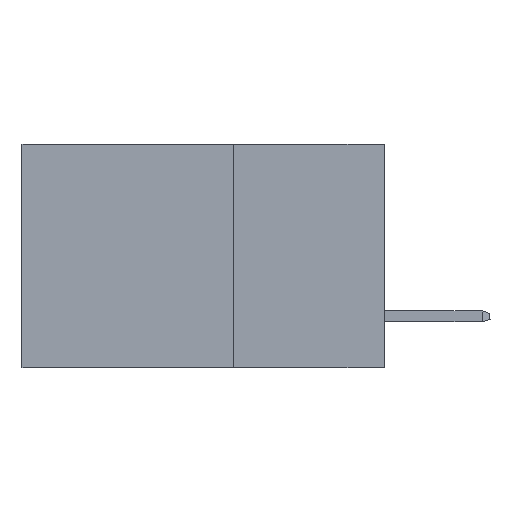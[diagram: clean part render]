
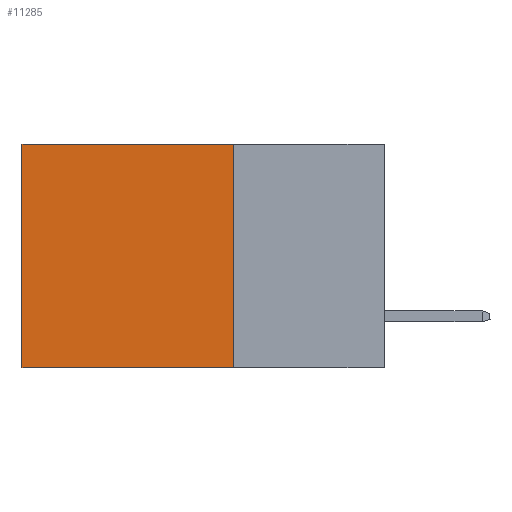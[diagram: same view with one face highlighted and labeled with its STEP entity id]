
A CAD part, left-side view. The second image highlights one B-rep face of the part: STEP entity #11285.
In plain terms, the highlighted planar face has unit normal (-1, 0, 0).
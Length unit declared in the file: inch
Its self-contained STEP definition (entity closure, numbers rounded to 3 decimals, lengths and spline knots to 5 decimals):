
#1179 = ORIENTED_EDGE ( 'NONE', *, *, #7643, .F. ) ;
#1474 = EDGE_CURVE ( 'NONE', #23829, #23262, #9127, .T. ) ;
#2188 = CARTESIAN_POINT ( 'NONE',  ( 0.2615, 0.6, 0. ) ) ;
#2611 = LINE ( 'NONE', #17897, #23378 ) ;
#3363 = DIRECTION ( 'NONE',  ( 0., 0., -1. ) ) ;
#6146 = DIRECTION ( 'NONE',  ( 0., 0., -1. ) ) ;
#7643 = EDGE_CURVE ( 'NONE', #25616, #23262, #22868, .T. ) ;
#8002 = DIRECTION ( 'NONE',  ( 0., 1., 0. ) ) ;
#8077 = CARTESIAN_POINT ( 'NONE',  ( 0.2615, 0.25, -0.37 ) ) ;
#8276 = CARTESIAN_POINT ( 'NONE',  ( 0.2615, 0.6, -0.37 ) ) ;
#9127 = LINE ( 'NONE', #19119, #25031 ) ;
#10938 = CARTESIAN_POINT ( 'NONE',  ( 0.2615, 0.25, -0.37 ) ) ;
#10996 = CARTESIAN_POINT ( 'NONE',  ( 0.2615, 0.25, 0. ) ) ;
#11285 = ADVANCED_FACE ( 'NONE', ( #23899 ), #14159, .F. ) ;
#11448 = CARTESIAN_POINT ( 'NONE',  ( 0.2615, 0.25, -0.37 ) ) ;
#11860 = AXIS2_PLACEMENT_3D ( 'NONE', #8077, #18147, #6146 ) ;
#12409 = DIRECTION ( 'NONE',  ( 0., 1., 0. ) ) ;
#12574 = CARTESIAN_POINT ( 'NONE',  ( 0.2615, 0.25, -0.37 ) ) ;
#12931 = LINE ( 'NONE', #11448, #22915 ) ;
#13049 = EDGE_CURVE ( 'NONE', #24311, #23829, #2611, .T. ) ;
#14060 = ORIENTED_EDGE ( 'NONE', *, *, #1474, .T. ) ;
#14159 = PLANE ( 'NONE',  #11860 ) ;
#17518 = VECTOR ( 'NONE', #12409, 39.37008 ) ;
#17739 = EDGE_LOOP ( 'NONE', ( #14060, #1179, #20037, #19972 ) ) ;
#17897 = CARTESIAN_POINT ( 'NONE',  ( 0.2615, 0.25, 0. ) ) ;
#18147 = DIRECTION ( 'NONE',  ( 1., 0., 0. ) ) ;
#19119 = CARTESIAN_POINT ( 'NONE',  ( 0.2615, 0.6, -0.37 ) ) ;
#19145 = DIRECTION ( 'NONE',  ( 0., 0., -1. ) ) ;
#19972 = ORIENTED_EDGE ( 'NONE', *, *, #13049, .T. ) ;
#20037 = ORIENTED_EDGE ( 'NONE', *, *, #23565, .F. ) ;
#22868 = LINE ( 'NONE', #12574, #17518 ) ;
#22915 = VECTOR ( 'NONE', #3363, 39.37008 ) ;
#23262 = VERTEX_POINT ( 'NONE', #8276 ) ;
#23378 = VECTOR ( 'NONE', #8002, 39.37008 ) ;
#23565 = EDGE_CURVE ( 'NONE', #24311, #25616, #12931, .T. ) ;
#23829 = VERTEX_POINT ( 'NONE', #2188 ) ;
#23899 = FACE_OUTER_BOUND ( 'NONE', #17739, .T. ) ;
#24311 = VERTEX_POINT ( 'NONE', #10996 ) ;
#25031 = VECTOR ( 'NONE', #19145, 39.37008 ) ;
#25616 = VERTEX_POINT ( 'NONE', #10938 ) ;
